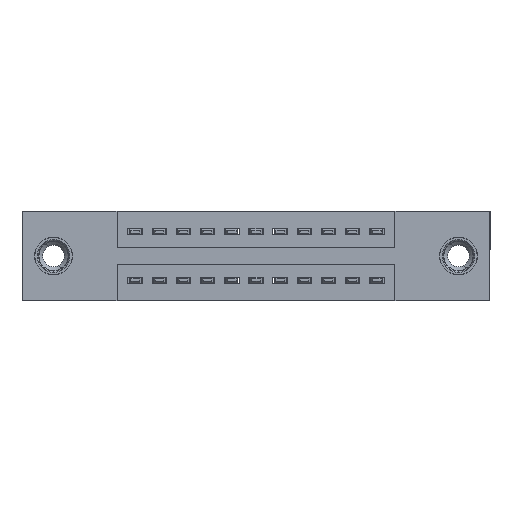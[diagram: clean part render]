
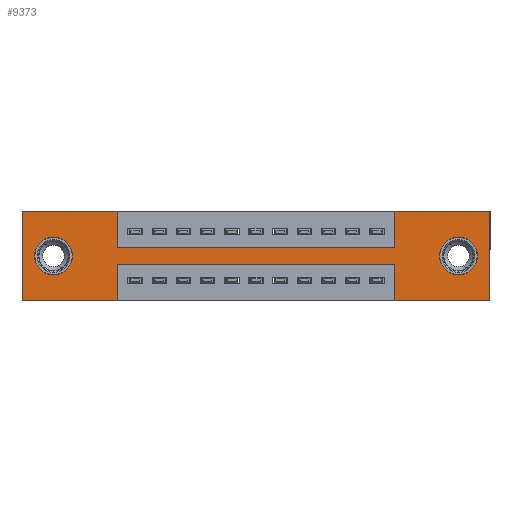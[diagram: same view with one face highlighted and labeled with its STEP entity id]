
A CAD part, front view. The second image highlights one B-rep face of the part: STEP entity #9373.
In plain terms, the highlighted planar face has unit normal (0, -1, 0).
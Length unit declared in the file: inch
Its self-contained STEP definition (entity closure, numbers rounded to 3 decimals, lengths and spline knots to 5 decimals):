
#39 = VERTEX_POINT ( 'NONE', #1813 ) ;
#101 = ORIENTED_EDGE ( 'NONE', *, *, #9736, .T. ) ;
#126 = DIRECTION ( 'NONE',  ( 0., 0., -1. ) ) ;
#436 = LINE ( 'NONE', #443, #5992 ) ;
#440 = CARTESIAN_POINT ( 'NONE',  ( 0.13, 0., -0.185 ) ) ;
#443 = CARTESIAN_POINT ( 'NONE',  ( 0.3925, 0., -0.22 ) ) ;
#448 = ORIENTED_EDGE ( 'NONE', *, *, #2200, .T. ) ;
#595 = VECTOR ( 'NONE', #2175, 39.37008 ) ;
#668 = EDGE_CURVE ( 'NONE', #11433, #10553, #9998, .T. ) ;
#726 = CARTESIAN_POINT ( 'NONE',  ( 1.5425, 0., -0.15 ) ) ;
#771 = VECTOR ( 'NONE', #11411, 39.37008 ) ;
#818 = DIRECTION ( 'NONE',  ( 0., 1., 0. ) ) ;
#869 = CIRCLE ( 'NONE', #13673, 0.078 ) ;
#976 = DIRECTION ( 'NONE',  ( 0., 0., -1. ) ) ;
#1044 = CARTESIAN_POINT ( 'NONE',  ( 0., 0., -0.37 ) ) ;
#1163 = EDGE_CURVE ( 'NONE', #13876, #2676, #4749, .T. ) ;
#1193 = DIRECTION ( 'NONE',  ( 0., 1., 0. ) ) ;
#1524 = VECTOR ( 'NONE', #12847, 39.37008 ) ;
#1531 = ORIENTED_EDGE ( 'NONE', *, *, #13110, .F. ) ;
#1566 = DIRECTION ( 'NONE',  ( 0., 0., 1. ) ) ;
#1645 = DIRECTION ( 'NONE',  ( 0., 0., 1. ) ) ;
#1654 = CIRCLE ( 'NONE', #6601, 0.078 ) ;
#1813 = CARTESIAN_POINT ( 'NONE',  ( 0.3925, 0., -0.37 ) ) ;
#1841 = CARTESIAN_POINT ( 'NONE',  ( 0., 0., 0. ) ) ;
#1891 = VECTOR ( 'NONE', #12114, 39.37008 ) ;
#1947 = LINE ( 'NONE', #9061, #7374 ) ;
#2145 = DIRECTION ( 'NONE',  ( -1., 0., 0. ) ) ;
#2175 = DIRECTION ( 'NONE',  ( 1., 0., 0. ) ) ;
#2200 = EDGE_CURVE ( 'NONE', #5719, #9779, #6009, .T. ) ;
#2302 = VERTEX_POINT ( 'NONE', #13789 ) ;
#2591 = EDGE_LOOP ( 'NONE', ( #101, #2631 ) ) ;
#2631 = ORIENTED_EDGE ( 'NONE', *, *, #4394, .T. ) ;
#2676 = VERTEX_POINT ( 'NONE', #8142 ) ;
#2840 = LINE ( 'NONE', #1841, #14471 ) ;
#2868 = ORIENTED_EDGE ( 'NONE', *, *, #7087, .F. ) ;
#2870 = CARTESIAN_POINT ( 'NONE',  ( 1.935, 0., 0. ) ) ;
#2943 = ORIENTED_EDGE ( 'NONE', *, *, #11856, .F. ) ;
#3166 = DIRECTION ( 'NONE',  ( 1., 0., 0. ) ) ;
#3512 = CARTESIAN_POINT ( 'NONE',  ( 0.3925, 0., -0.15 ) ) ;
#3732 = ORIENTED_EDGE ( 'NONE', *, *, #11332, .T. ) ;
#3942 = VERTEX_POINT ( 'NONE', #9339 ) ;
#4339 = LINE ( 'NONE', #7738, #12918 ) ;
#4378 = CARTESIAN_POINT ( 'NONE',  ( 1.5425, 0., -0.37 ) ) ;
#4394 = EDGE_CURVE ( 'NONE', #10695, #7702, #869, .T. ) ;
#4724 = VECTOR ( 'NONE', #14104, 39.37008 ) ;
#4749 = LINE ( 'NONE', #4378, #12618 ) ;
#5176 = ORIENTED_EDGE ( 'NONE', *, *, #6831, .F. ) ;
#5250 = CARTESIAN_POINT ( 'NONE',  ( 0.3925, 0., 0. ) ) ;
#5394 = AXIS2_PLACEMENT_3D ( 'NONE', #5684, #7931, #976 ) ;
#5433 = DIRECTION ( 'NONE',  ( 0., 1., 0. ) ) ;
#5480 = CARTESIAN_POINT ( 'NONE',  ( 1.805, 0., -0.185 ) ) ;
#5684 = CARTESIAN_POINT ( 'NONE',  ( 0., 0., -0.37 ) ) ;
#5698 = CARTESIAN_POINT ( 'NONE',  ( 0.13, 0., -0.263 ) ) ;
#5719 = VERTEX_POINT ( 'NONE', #6917 ) ;
#5887 = FACE_BOUND ( 'NONE', #2591, .T. ) ;
#5992 = VECTOR ( 'NONE', #8576, 39.37008 ) ;
#6009 = CIRCLE ( 'NONE', #7841, 0.078 ) ;
#6134 = CARTESIAN_POINT ( 'NONE',  ( 1.935, 0., 0. ) ) ;
#6272 = VECTOR ( 'NONE', #2145, 39.37008 ) ;
#6601 = AXIS2_PLACEMENT_3D ( 'NONE', #440, #8573, #1645 ) ;
#6616 = DIRECTION ( 'NONE',  ( 0., 0., 1. ) ) ;
#6831 = EDGE_CURVE ( 'NONE', #9495, #13861, #12805, .T. ) ;
#6836 = ORIENTED_EDGE ( 'NONE', *, *, #668, .F. ) ;
#6876 = VERTEX_POINT ( 'NONE', #1044 ) ;
#6917 = CARTESIAN_POINT ( 'NONE',  ( 1.805, 0., -0.263 ) ) ;
#7087 = EDGE_CURVE ( 'NONE', #13861, #2302, #9643, .T. ) ;
#7374 = VECTOR ( 'NONE', #11321, 39.37008 ) ;
#7425 = CARTESIAN_POINT ( 'NONE',  ( 0.3925, 0., 0. ) ) ;
#7463 = CARTESIAN_POINT ( 'NONE',  ( 1.5425, 0., -0.37 ) ) ;
#7597 = EDGE_LOOP ( 'NONE', ( #3732, #448 ) ) ;
#7702 = VERTEX_POINT ( 'NONE', #9609 ) ;
#7738 = CARTESIAN_POINT ( 'NONE',  ( 1.5425, 0., 0. ) ) ;
#7778 = CARTESIAN_POINT ( 'NONE',  ( 0.13, 0., -0.185 ) ) ;
#7784 = VERTEX_POINT ( 'NONE', #5250 ) ;
#7841 = AXIS2_PLACEMENT_3D ( 'NONE', #5480, #5433, #126 ) ;
#7853 = EDGE_CURVE ( 'NONE', #3942, #39, #11021, .T. ) ;
#7882 = ORIENTED_EDGE ( 'NONE', *, *, #7853, .F. ) ;
#7931 = DIRECTION ( 'NONE',  ( 0., -1., 0. ) ) ;
#7967 = EDGE_CURVE ( 'NONE', #39, #6876, #9276, .T. ) ;
#8068 = DIRECTION ( 'NONE',  ( -1., 0., 0. ) ) ;
#8139 = CARTESIAN_POINT ( 'NONE',  ( 1.805, 0., -0.185 ) ) ;
#8142 = CARTESIAN_POINT ( 'NONE',  ( 1.5425, 0., -0.22 ) ) ;
#8373 = EDGE_CURVE ( 'NONE', #7784, #11433, #10649, .T. ) ;
#8538 = EDGE_CURVE ( 'NONE', #13280, #7784, #2840, .T. ) ;
#8573 = DIRECTION ( 'NONE',  ( 0., 1., 0. ) ) ;
#8576 = DIRECTION ( 'NONE',  ( -1., 0., 0. ) ) ;
#8619 = ORIENTED_EDGE ( 'NONE', *, *, #11549, .F. ) ;
#8866 = FACE_BOUND ( 'NONE', #7597, .T. ) ;
#8924 = DIRECTION ( 'NONE',  ( 0., 0., 1. ) ) ;
#9021 = ORIENTED_EDGE ( 'NONE', *, *, #8538, .F. ) ;
#9061 = CARTESIAN_POINT ( 'NONE',  ( 0., 0., 0. ) ) ;
#9167 = ORIENTED_EDGE ( 'NONE', *, *, #1163, .F. ) ;
#9276 = LINE ( 'NONE', #13445, #6272 ) ;
#9281 = DIRECTION ( 'NONE',  ( 0., 0., -1. ) ) ;
#9339 = CARTESIAN_POINT ( 'NONE',  ( 0.3925, 0., -0.22 ) ) ;
#9373 = ADVANCED_FACE ( 'NONE', ( #8866, #5887, #11848 ), #13513, .T. ) ;
#9495 = VERTEX_POINT ( 'NONE', #12661 ) ;
#9609 = CARTESIAN_POINT ( 'NONE',  ( 0.13, 0., -0.107 ) ) ;
#9643 = LINE ( 'NONE', #6134, #1524 ) ;
#9736 = EDGE_CURVE ( 'NONE', #7702, #10695, #1654, .T. ) ;
#9779 = VERTEX_POINT ( 'NONE', #13122 ) ;
#9998 = LINE ( 'NONE', #3512, #771 ) ;
#10168 = CARTESIAN_POINT ( 'NONE',  ( 0., 0., 0. ) ) ;
#10488 = AXIS2_PLACEMENT_3D ( 'NONE', #8139, #1193, #9281 ) ;
#10553 = VERTEX_POINT ( 'NONE', #726 ) ;
#10649 = LINE ( 'NONE', #7425, #4724 ) ;
#10670 = VECTOR ( 'NONE', #8068, 39.37008 ) ;
#10695 = VERTEX_POINT ( 'NONE', #5698 ) ;
#10973 = CARTESIAN_POINT ( 'NONE',  ( 0.3925, 0., -0.37 ) ) ;
#11021 = LINE ( 'NONE', #10973, #1891 ) ;
#11085 = ORIENTED_EDGE ( 'NONE', *, *, #7967, .F. ) ;
#11321 = DIRECTION ( 'NONE',  ( 0., 0., 1. ) ) ;
#11332 = EDGE_CURVE ( 'NONE', #9779, #5719, #14172, .T. ) ;
#11411 = DIRECTION ( 'NONE',  ( 1., 0., 0. ) ) ;
#11433 = VERTEX_POINT ( 'NONE', #13841 ) ;
#11549 = EDGE_CURVE ( 'NONE', #2676, #3942, #436, .T. ) ;
#11696 = CARTESIAN_POINT ( 'NONE',  ( 0., 0., 0. ) ) ;
#11848 = FACE_OUTER_BOUND ( 'NONE', #12860, .T. ) ;
#11856 = EDGE_CURVE ( 'NONE', #6876, #13280, #1947, .T. ) ;
#12114 = DIRECTION ( 'NONE',  ( 0., 0., -1. ) ) ;
#12618 = VECTOR ( 'NONE', #1566, 39.37008 ) ;
#12661 = CARTESIAN_POINT ( 'NONE',  ( 1.5425, 0., 0. ) ) ;
#12765 = ORIENTED_EDGE ( 'NONE', *, *, #8373, .F. ) ;
#12805 = LINE ( 'NONE', #10168, #595 ) ;
#12836 = ORIENTED_EDGE ( 'NONE', *, *, #14052, .F. ) ;
#12847 = DIRECTION ( 'NONE',  ( 0., 0., -1. ) ) ;
#12860 = EDGE_LOOP ( 'NONE', ( #7882, #8619, #9167, #1531, #2868, #5176, #12836, #6836, #12765, #9021, #2943, #11085 ) ) ;
#12918 = VECTOR ( 'NONE', #6616, 39.37008 ) ;
#13110 = EDGE_CURVE ( 'NONE', #2302, #13876, #13969, .T. ) ;
#13122 = CARTESIAN_POINT ( 'NONE',  ( 1.805, 0., -0.107 ) ) ;
#13280 = VERTEX_POINT ( 'NONE', #11696 ) ;
#13445 = CARTESIAN_POINT ( 'NONE',  ( 0., 0., -0.37 ) ) ;
#13513 = PLANE ( 'NONE',  #5394 ) ;
#13673 = AXIS2_PLACEMENT_3D ( 'NONE', #7778, #818, #8924 ) ;
#13686 = CARTESIAN_POINT ( 'NONE',  ( 0., 0., -0.37 ) ) ;
#13789 = CARTESIAN_POINT ( 'NONE',  ( 1.935, 0., -0.37 ) ) ;
#13841 = CARTESIAN_POINT ( 'NONE',  ( 0.3925, 0., -0.15 ) ) ;
#13861 = VERTEX_POINT ( 'NONE', #2870 ) ;
#13876 = VERTEX_POINT ( 'NONE', #7463 ) ;
#13969 = LINE ( 'NONE', #13686, #10670 ) ;
#14052 = EDGE_CURVE ( 'NONE', #10553, #9495, #4339, .T. ) ;
#14104 = DIRECTION ( 'NONE',  ( 0., 0., -1. ) ) ;
#14172 = CIRCLE ( 'NONE', #10488, 0.078 ) ;
#14471 = VECTOR ( 'NONE', #3166, 39.37008 ) ;
